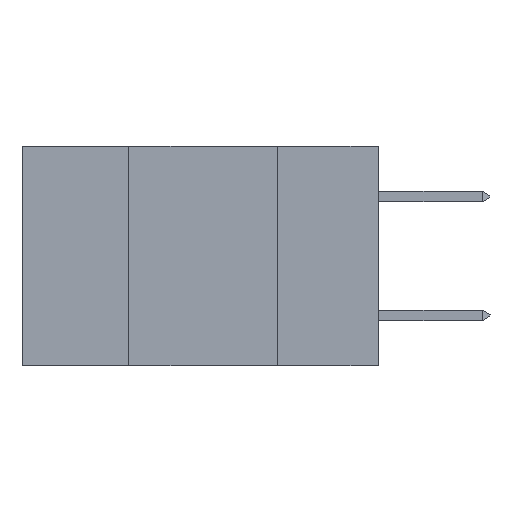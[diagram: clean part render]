
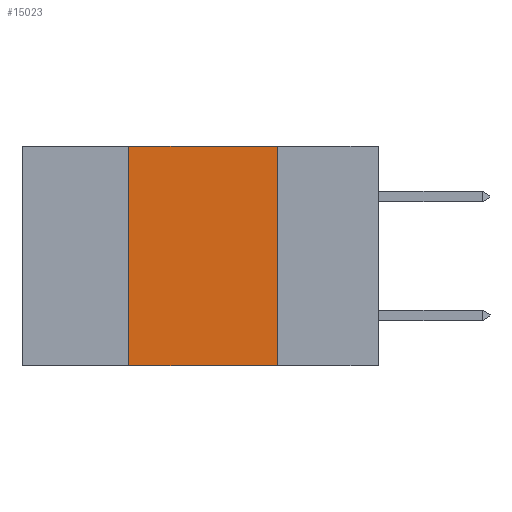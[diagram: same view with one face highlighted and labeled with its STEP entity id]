
A CAD part, left-side view. The second image highlights one B-rep face of the part: STEP entity #15023.
In plain terms, the highlighted planar face has unit normal (-1, 0, 0).
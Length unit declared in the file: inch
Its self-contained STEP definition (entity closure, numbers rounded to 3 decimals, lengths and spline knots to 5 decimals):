
#1151 = VECTOR ( 'NONE', #13840, 39.37008 ) ;
#1452 = CARTESIAN_POINT ( 'NONE',  ( 0., 0.17, 0. ) ) ;
#1630 = ORIENTED_EDGE ( 'NONE', *, *, #12858, .F. ) ;
#1948 = DIRECTION ( 'NONE',  ( 0., -1., 0. ) ) ;
#3278 = CARTESIAN_POINT ( 'NONE',  ( 0., 0.6, -0.37 ) ) ;
#7655 = CARTESIAN_POINT ( 'NONE',  ( 0., 0.17, 0. ) ) ;
#8172 = EDGE_CURVE ( 'NONE', #25232, #12924, #17204, .T. ) ;
#8196 = CARTESIAN_POINT ( 'NONE',  ( 0., 0.17, -0.37 ) ) ;
#8486 = CARTESIAN_POINT ( 'NONE',  ( 0., 0.6, 0. ) ) ;
#10605 = LINE ( 'NONE', #14711, #22611 ) ;
#10994 = LINE ( 'NONE', #1452, #26006 ) ;
#11365 = EDGE_CURVE ( 'NONE', #22975, #12924, #10994, .T. ) ;
#12498 = DIRECTION ( 'NONE',  ( 0., 0., 1. ) ) ;
#12526 = CARTESIAN_POINT ( 'NONE',  ( 0., 0.6, 0. ) ) ;
#12858 = EDGE_CURVE ( 'NONE', #25232, #21477, #10605, .T. ) ;
#12924 = VERTEX_POINT ( 'NONE', #8196 ) ;
#13641 = CARTESIAN_POINT ( 'NONE',  ( 0., 0.42, 0. ) ) ;
#13840 = DIRECTION ( 'NONE',  ( 0., -1., 0. ) ) ;
#14711 = CARTESIAN_POINT ( 'NONE',  ( 0., 0.42, 0. ) ) ;
#14861 = VECTOR ( 'NONE', #1948, 39.37008 ) ;
#15023 = ADVANCED_FACE ( 'NONE', ( #16562 ), #21245, .F. ) ;
#15397 = EDGE_CURVE ( 'NONE', #21477, #22975, #23221, .T. ) ;
#15664 = EDGE_LOOP ( 'NONE', ( #22087, #21566, #1630, #23936 ) ) ;
#16562 = FACE_OUTER_BOUND ( 'NONE', #15664, .T. ) ;
#17204 = LINE ( 'NONE', #3278, #1151 ) ;
#18824 = CARTESIAN_POINT ( 'NONE',  ( 0., 0.42, -0.37 ) ) ;
#20789 = DIRECTION ( 'NONE',  ( 0., 0., -1. ) ) ;
#21245 = PLANE ( 'NONE',  #23275 ) ;
#21477 = VERTEX_POINT ( 'NONE', #13641 ) ;
#21566 = ORIENTED_EDGE ( 'NONE', *, *, #15397, .F. ) ;
#22087 = ORIENTED_EDGE ( 'NONE', *, *, #11365, .F. ) ;
#22611 = VECTOR ( 'NONE', #12498, 39.37008 ) ;
#22975 = VERTEX_POINT ( 'NONE', #7655 ) ;
#23221 = LINE ( 'NONE', #12526, #14861 ) ;
#23275 = AXIS2_PLACEMENT_3D ( 'NONE', #8486, #23392, #23682 ) ;
#23392 = DIRECTION ( 'NONE',  ( 1., 0., 0. ) ) ;
#23682 = DIRECTION ( 'NONE',  ( 0., 0., -1. ) ) ;
#23936 = ORIENTED_EDGE ( 'NONE', *, *, #8172, .T. ) ;
#25232 = VERTEX_POINT ( 'NONE', #18824 ) ;
#26006 = VECTOR ( 'NONE', #20789, 39.37008 ) ;
